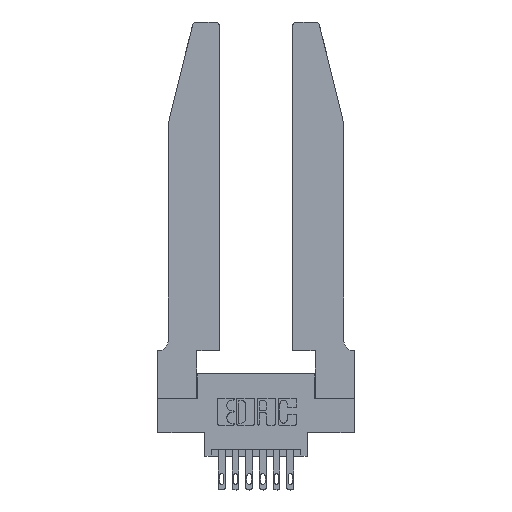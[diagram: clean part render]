
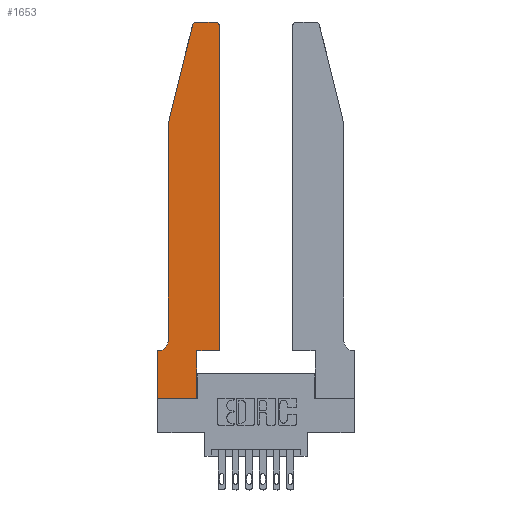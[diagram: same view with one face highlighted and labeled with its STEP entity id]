
A CAD part, top view. The second image highlights one B-rep face of the part: STEP entity #1653.
In plain terms, the highlighted planar face has unit normal (0, 0, 1).
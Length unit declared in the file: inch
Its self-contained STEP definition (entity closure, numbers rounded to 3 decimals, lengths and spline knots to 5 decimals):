
#76 = ORIENTED_EDGE ( 'NONE', *, *, #12508, .T. ) ;
#129 = VERTEX_POINT ( 'NONE', #8141 ) ;
#212 = AXIS2_PLACEMENT_3D ( 'NONE', #769, #14180, #9680 ) ;
#242 = LINE ( 'NONE', #8887, #10171 ) ;
#371 = VERTEX_POINT ( 'NONE', #4329 ) ;
#398 = CARTESIAN_POINT ( 'NONE',  ( 0.4505, 0.35, 0.37 ) ) ;
#715 = EDGE_CURVE ( 'NONE', #10280, #13728, #14375, .T. ) ;
#769 = CARTESIAN_POINT ( 'NONE',  ( 0.4205, 2.72, 0.37 ) ) ;
#932 = CARTESIAN_POINT ( 'NONE',  ( 0., 0., 0.37 ) ) ;
#1155 = LINE ( 'NONE', #2083, #3239 ) ;
#1325 = VECTOR ( 'NONE', #7358, 39.37008 ) ;
#1346 = CARTESIAN_POINT ( 'NONE',  ( 0.284, 2.75, 0.37 ) ) ;
#1373 = ORIENTED_EDGE ( 'NONE', *, *, #3059, .T. ) ;
#1422 = VERTEX_POINT ( 'NONE', #9392 ) ;
#1653 = ADVANCED_FACE ( 'NONE', ( #3726 ), #1853, .T. ) ;
#1703 = EDGE_CURVE ( 'NONE', #5193, #371, #2176, .T. ) ;
#1752 = CARTESIAN_POINT ( 'NONE',  ( 0., 0.35, 0.37 ) ) ;
#1853 = PLANE ( 'NONE',  #3608 ) ;
#1902 = DIRECTION ( 'NONE',  ( 0., 1., 0. ) ) ;
#2007 = CARTESIAN_POINT ( 'NONE',  ( 0.284, 2.72, 0.37 ) ) ;
#2083 = CARTESIAN_POINT ( 'NONE',  ( 0., 0., 0.37 ) ) ;
#2176 = CIRCLE ( 'NONE', #7935, 0.07 ) ;
#2722 = ORIENTED_EDGE ( 'NONE', *, *, #1703, .T. ) ;
#2836 = LINE ( 'NONE', #9816, #8082 ) ;
#3059 = EDGE_CURVE ( 'NONE', #5113, #6565, #14296, .T. ) ;
#3105 = VECTOR ( 'NONE', #14003, 39.37008 ) ;
#3165 = EDGE_CURVE ( 'NONE', #129, #7658, #2836, .T. ) ;
#3239 = VECTOR ( 'NONE', #12584, 39.37008 ) ;
#3407 = CARTESIAN_POINT ( 'NONE',  ( 0.25487, 2.72718, 0.37 ) ) ;
#3485 = ORIENTED_EDGE ( 'NONE', *, *, #5092, .T. ) ;
#3570 = AXIS2_PLACEMENT_3D ( 'NONE', #2007, #8542, #5246 ) ;
#3608 = AXIS2_PLACEMENT_3D ( 'NONE', #1752, #11846, #10807 ) ;
#3726 = FACE_OUTER_BOUND ( 'NONE', #10710, .T. ) ;
#3816 = ORIENTED_EDGE ( 'NONE', *, *, #6631, .T. ) ;
#4177 = CARTESIAN_POINT ( 'NONE',  ( 0.2865, 0.35, 0.37 ) ) ;
#4282 = DIRECTION ( 'NONE',  ( -1., 0., 0. ) ) ;
#4297 = DIRECTION ( 'NONE',  ( 0., 1., 0. ) ) ;
#4329 = CARTESIAN_POINT ( 'NONE',  ( 0.0055, 0.35, 0.37 ) ) ;
#4400 = CARTESIAN_POINT ( 'NONE',  ( 0.4505, 0.35, 0.37 ) ) ;
#4662 = CIRCLE ( 'NONE', #212, 0.03 ) ;
#5092 = EDGE_CURVE ( 'NONE', #13728, #5193, #11818, .T. ) ;
#5107 = CARTESIAN_POINT ( 'NONE',  ( 0.2865, 0., 0.37 ) ) ;
#5113 = VERTEX_POINT ( 'NONE', #398 ) ;
#5193 = VERTEX_POINT ( 'NONE', #11437 ) ;
#5246 = DIRECTION ( 'NONE',  ( 1., 0., 0. ) ) ;
#6325 = CARTESIAN_POINT ( 'NONE',  ( 0.2865, 0.35, 0.37 ) ) ;
#6453 = DIRECTION ( 'NONE',  ( -1., 0., 0. ) ) ;
#6565 = VERTEX_POINT ( 'NONE', #7780 ) ;
#6631 = EDGE_CURVE ( 'NONE', #371, #1422, #242, .T. ) ;
#6719 = ORIENTED_EDGE ( 'NONE', *, *, #10061, .T. ) ;
#6838 = EDGE_CURVE ( 'NONE', #11273, #5113, #12377, .T. ) ;
#7323 = EDGE_CURVE ( 'NONE', #9727, #11273, #8589, .T. ) ;
#7358 = DIRECTION ( 'NONE',  ( -0.239, -0.971, 0. ) ) ;
#7658 = VERTEX_POINT ( 'NONE', #1346 ) ;
#7664 = DIRECTION ( 'NONE',  ( 0., 0., -1. ) ) ;
#7780 = CARTESIAN_POINT ( 'NONE',  ( 0.4505, 2.72, 0.37 ) ) ;
#7935 = AXIS2_PLACEMENT_3D ( 'NONE', #12798, #7664, #10947 ) ;
#8082 = VECTOR ( 'NONE', #6453, 39.37008 ) ;
#8088 = ORIENTED_EDGE ( 'NONE', *, *, #3165, .T. ) ;
#8141 = CARTESIAN_POINT ( 'NONE',  ( 0.4205, 2.75, 0.37 ) ) ;
#8152 = ORIENTED_EDGE ( 'NONE', *, *, #715, .T. ) ;
#8192 = LINE ( 'NONE', #12711, #3105 ) ;
#8471 = CIRCLE ( 'NONE', #3570, 0.03 ) ;
#8542 = DIRECTION ( 'NONE',  ( 0., 0., 1. ) ) ;
#8589 = LINE ( 'NONE', #6325, #11187 ) ;
#8650 = CARTESIAN_POINT ( 'NONE',  ( 0.4505, 0.35, 0.37 ) ) ;
#8763 = VECTOR ( 'NONE', #4297, 39.37008 ) ;
#8887 = CARTESIAN_POINT ( 'NONE',  ( 0.0755, 0.35, 0.37 ) ) ;
#8909 = VECTOR ( 'NONE', #10381, 39.37008 ) ;
#9150 = ORIENTED_EDGE ( 'NONE', *, *, #10748, .T. ) ;
#9392 = CARTESIAN_POINT ( 'NONE',  ( 0., 0.35, 0.37 ) ) ;
#9680 = DIRECTION ( 'NONE',  ( 1., 0., 0. ) ) ;
#9714 = ORIENTED_EDGE ( 'NONE', *, *, #6838, .T. ) ;
#9727 = VERTEX_POINT ( 'NONE', #5107 ) ;
#9816 = CARTESIAN_POINT ( 'NONE',  ( 0.2605, 2.75, 0.37 ) ) ;
#9872 = VERTEX_POINT ( 'NONE', #932 ) ;
#10061 = EDGE_CURVE ( 'NONE', #6565, #129, #4662, .T. ) ;
#10157 = CARTESIAN_POINT ( 'NONE',  ( 0.0755, 2., 0.37 ) ) ;
#10171 = VECTOR ( 'NONE', #4282, 39.37008 ) ;
#10280 = VERTEX_POINT ( 'NONE', #3407 ) ;
#10330 = CARTESIAN_POINT ( 'NONE',  ( 0.0755, 2., 0.37 ) ) ;
#10381 = DIRECTION ( 'NONE',  ( 0., -1., 0. ) ) ;
#10710 = EDGE_LOOP ( 'NONE', ( #8088, #76, #8152, #3485, #2722, #3816, #9150, #12466, #13815, #9714, #1373, #6719 ) ) ;
#10748 = EDGE_CURVE ( 'NONE', #1422, #9872, #8192, .T. ) ;
#10807 = DIRECTION ( 'NONE',  ( 1., 0., 0. ) ) ;
#10947 = DIRECTION ( 'NONE',  ( -1., 0., 0. ) ) ;
#11187 = VECTOR ( 'NONE', #1902, 39.37008 ) ;
#11273 = VERTEX_POINT ( 'NONE', #4177 ) ;
#11437 = CARTESIAN_POINT ( 'NONE',  ( 0.0755, 0.42, 0.37 ) ) ;
#11661 = CARTESIAN_POINT ( 'NONE',  ( 0.0755, 2., 0.37 ) ) ;
#11818 = LINE ( 'NONE', #10330, #8909 ) ;
#11846 = DIRECTION ( 'NONE',  ( 0., 0., 1. ) ) ;
#12182 = DIRECTION ( 'NONE',  ( 1., 0., 0. ) ) ;
#12377 = LINE ( 'NONE', #4400, #12554 ) ;
#12466 = ORIENTED_EDGE ( 'NONE', *, *, #13587, .T. ) ;
#12508 = EDGE_CURVE ( 'NONE', #7658, #10280, #8471, .T. ) ;
#12554 = VECTOR ( 'NONE', #12182, 39.37008 ) ;
#12584 = DIRECTION ( 'NONE',  ( 1., 0., 0. ) ) ;
#12711 = CARTESIAN_POINT ( 'NONE',  ( 0., 0., 0.37 ) ) ;
#12798 = CARTESIAN_POINT ( 'NONE',  ( 0.0055, 0.42, 0.37 ) ) ;
#13587 = EDGE_CURVE ( 'NONE', #9872, #9727, #1155, .T. ) ;
#13728 = VERTEX_POINT ( 'NONE', #10157 ) ;
#13815 = ORIENTED_EDGE ( 'NONE', *, *, #7323, .T. ) ;
#14003 = DIRECTION ( 'NONE',  ( 0., -1., 0. ) ) ;
#14180 = DIRECTION ( 'NONE',  ( 0., 0., 1. ) ) ;
#14296 = LINE ( 'NONE', #8650, #8763 ) ;
#14375 = LINE ( 'NONE', #11661, #1325 ) ;
